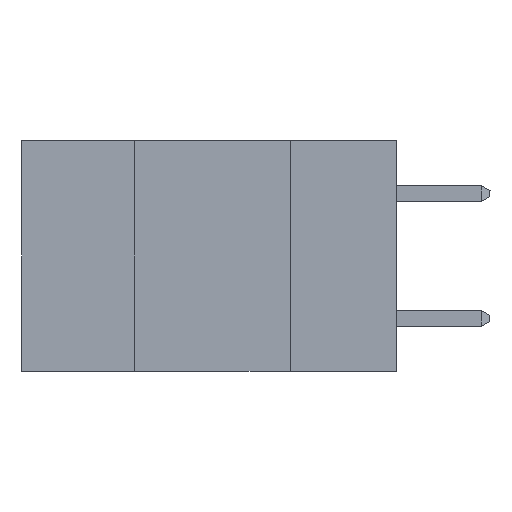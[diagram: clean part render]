
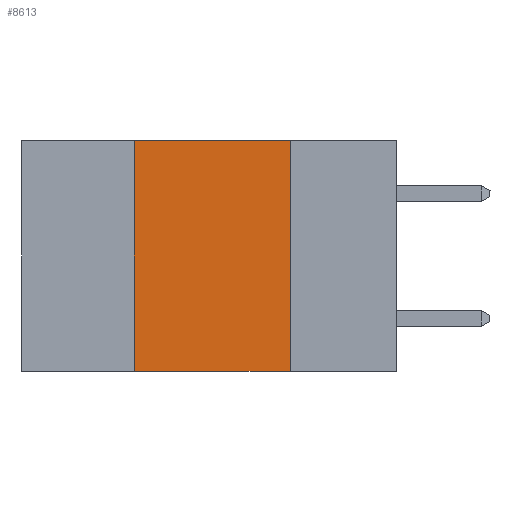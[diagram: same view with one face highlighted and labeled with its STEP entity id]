
A CAD part, left-side view. The second image highlights one B-rep face of the part: STEP entity #8613.
In plain terms, the highlighted planar face has unit normal (-1, 0, 0).
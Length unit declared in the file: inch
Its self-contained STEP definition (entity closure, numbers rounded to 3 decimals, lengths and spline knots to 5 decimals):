
#173 = CARTESIAN_POINT ( 'NONE',  ( 0., 0.42, 0. ) ) ;
#376 = ORIENTED_EDGE ( 'NONE', *, *, #5563, .F. ) ;
#645 = ORIENTED_EDGE ( 'NONE', *, *, #5828, .T. ) ;
#1066 = CARTESIAN_POINT ( 'NONE',  ( 0., 0.17, -0.37 ) ) ;
#1089 = CARTESIAN_POINT ( 'NONE',  ( 0., 0.42, 0. ) ) ;
#1311 = VERTEX_POINT ( 'NONE', #173 ) ;
#1429 = VECTOR ( 'NONE', #9282, 39.37008 ) ;
#1954 = DIRECTION ( 'NONE',  ( 0., 0., -1. ) ) ;
#2137 = LINE ( 'NONE', #1089, #5810 ) ;
#2415 = ORIENTED_EDGE ( 'NONE', *, *, #5466, .F. ) ;
#2482 = AXIS2_PLACEMENT_3D ( 'NONE', #7948, #7614, #1954 ) ;
#2519 = EDGE_LOOP ( 'NONE', ( #6105, #376, #2415, #645 ) ) ;
#2585 = VECTOR ( 'NONE', #8785, 39.37008 ) ;
#2641 = VERTEX_POINT ( 'NONE', #5623 ) ;
#2845 = LINE ( 'NONE', #8804, #6699 ) ;
#3102 = DIRECTION ( 'NONE',  ( 0., 0., -1. ) ) ;
#3377 = VERTEX_POINT ( 'NONE', #8907 ) ;
#3596 = CARTESIAN_POINT ( 'NONE',  ( 0., 0.6, -0.37 ) ) ;
#5135 = LINE ( 'NONE', #8412, #1429 ) ;
#5336 = EDGE_CURVE ( 'NONE', #2641, #9453, #2845, .T. ) ;
#5466 = EDGE_CURVE ( 'NONE', #3377, #1311, #2137, .T. ) ;
#5563 = EDGE_CURVE ( 'NONE', #1311, #2641, #5135, .T. ) ;
#5623 = CARTESIAN_POINT ( 'NONE',  ( 0., 0.17, 0. ) ) ;
#5810 = VECTOR ( 'NONE', #8647, 39.37008 ) ;
#5828 = EDGE_CURVE ( 'NONE', #3377, #9453, #8388, .T. ) ;
#6105 = ORIENTED_EDGE ( 'NONE', *, *, #5336, .F. ) ;
#6192 = PLANE ( 'NONE',  #2482 ) ;
#6699 = VECTOR ( 'NONE', #3102, 39.37008 ) ;
#7614 = DIRECTION ( 'NONE',  ( 1., 0., 0. ) ) ;
#7948 = CARTESIAN_POINT ( 'NONE',  ( 0., 0.6, 0. ) ) ;
#8388 = LINE ( 'NONE', #3596, #2585 ) ;
#8412 = CARTESIAN_POINT ( 'NONE',  ( 0., 0.6, 0. ) ) ;
#8613 = ADVANCED_FACE ( 'NONE', ( #8784 ), #6192, .F. ) ;
#8647 = DIRECTION ( 'NONE',  ( 0., 0., 1. ) ) ;
#8784 = FACE_OUTER_BOUND ( 'NONE', #2519, .T. ) ;
#8785 = DIRECTION ( 'NONE',  ( 0., -1., 0. ) ) ;
#8804 = CARTESIAN_POINT ( 'NONE',  ( 0., 0.17, 0. ) ) ;
#8907 = CARTESIAN_POINT ( 'NONE',  ( 0., 0.42, -0.37 ) ) ;
#9282 = DIRECTION ( 'NONE',  ( 0., -1., 0. ) ) ;
#9453 = VERTEX_POINT ( 'NONE', #1066 ) ;
